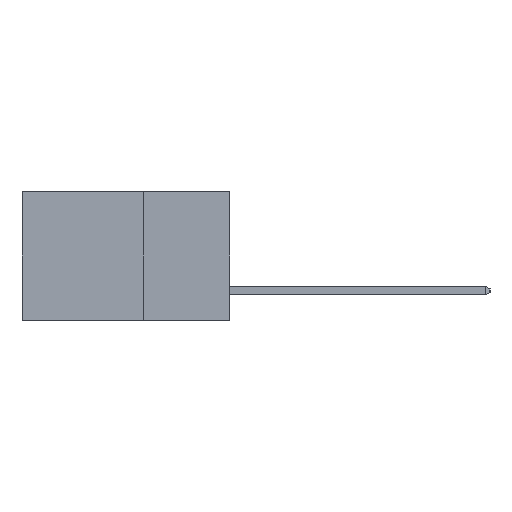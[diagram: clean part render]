
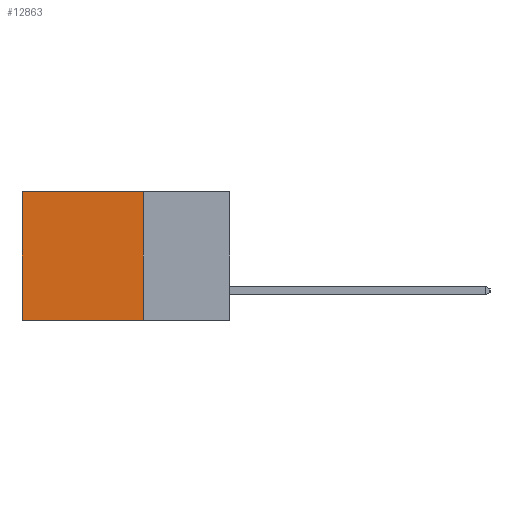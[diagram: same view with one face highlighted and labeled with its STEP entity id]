
A CAD part, left-side view. The second image highlights one B-rep face of the part: STEP entity #12863.
In plain terms, the highlighted planar face has unit normal (-1, 0, 0).
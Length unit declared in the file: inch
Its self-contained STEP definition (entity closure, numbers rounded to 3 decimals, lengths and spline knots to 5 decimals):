
#165 = LINE ( 'NONE', #19291, #19739 ) ;
#194 = CARTESIAN_POINT ( 'NONE',  ( 0.298, 0.25, -0.37 ) ) ;
#925 = VERTEX_POINT ( 'NONE', #18701 ) ;
#1509 = DIRECTION ( 'NONE',  ( 0., 0., -1. ) ) ;
#2075 = DIRECTION ( 'NONE',  ( 0., 1., 0. ) ) ;
#2115 = CARTESIAN_POINT ( 'NONE',  ( 0.298, 0.6, 0. ) ) ;
#2345 = VERTEX_POINT ( 'NONE', #23334 ) ;
#3007 = ORIENTED_EDGE ( 'NONE', *, *, #11482, .T. ) ;
#3818 = LINE ( 'NONE', #194, #13405 ) ;
#4453 = EDGE_CURVE ( 'NONE', #2345, #9066, #16825, .T. ) ;
#6344 = PLANE ( 'NONE',  #22589 ) ;
#6988 = FACE_OUTER_BOUND ( 'NONE', #13480, .T. ) ;
#9066 = VERTEX_POINT ( 'NONE', #2115 ) ;
#9862 = DIRECTION ( 'NONE',  ( 0., 1., 0. ) ) ;
#10225 = DIRECTION ( 'NONE',  ( 0., 0., -1. ) ) ;
#11085 = ORIENTED_EDGE ( 'NONE', *, *, #11086, .F. ) ;
#11086 = EDGE_CURVE ( 'NONE', #2345, #925, #165, .T. ) ;
#11113 = CARTESIAN_POINT ( 'NONE',  ( 0.298, 0.6, 0. ) ) ;
#11482 = EDGE_CURVE ( 'NONE', #9066, #13615, #14767, .T. ) ;
#12863 = ADVANCED_FACE ( 'NONE', ( #6988 ), #6344, .F. ) ;
#12869 = ORIENTED_EDGE ( 'NONE', *, *, #4453, .T. ) ;
#13405 = VECTOR ( 'NONE', #2075, 39.37008 ) ;
#13480 = EDGE_LOOP ( 'NONE', ( #3007, #16022, #11085, #12869 ) ) ;
#13615 = VERTEX_POINT ( 'NONE', #16055 ) ;
#14767 = LINE ( 'NONE', #11113, #24064 ) ;
#15628 = EDGE_CURVE ( 'NONE', #925, #13615, #3818, .T. ) ;
#16022 = ORIENTED_EDGE ( 'NONE', *, *, #15628, .F. ) ;
#16055 = CARTESIAN_POINT ( 'NONE',  ( 0.298, 0.6, -0.37 ) ) ;
#16241 = VECTOR ( 'NONE', #9862, 39.37008 ) ;
#16825 = LINE ( 'NONE', #23814, #16241 ) ;
#18701 = CARTESIAN_POINT ( 'NONE',  ( 0.298, 0.25, -0.37 ) ) ;
#19291 = CARTESIAN_POINT ( 'NONE',  ( 0.298, 0.25, 0. ) ) ;
#19555 = CARTESIAN_POINT ( 'NONE',  ( 0.298, 0.25, 0. ) ) ;
#19739 = VECTOR ( 'NONE', #21171, 39.37008 ) ;
#21171 = DIRECTION ( 'NONE',  ( 0., 0., -1. ) ) ;
#21435 = DIRECTION ( 'NONE',  ( 1., 0., 0. ) ) ;
#22589 = AXIS2_PLACEMENT_3D ( 'NONE', #19555, #21435, #10225 ) ;
#23334 = CARTESIAN_POINT ( 'NONE',  ( 0.298, 0.25, 0. ) ) ;
#23814 = CARTESIAN_POINT ( 'NONE',  ( 0.298, 0.25, 0. ) ) ;
#24064 = VECTOR ( 'NONE', #1509, 39.37008 ) ;
